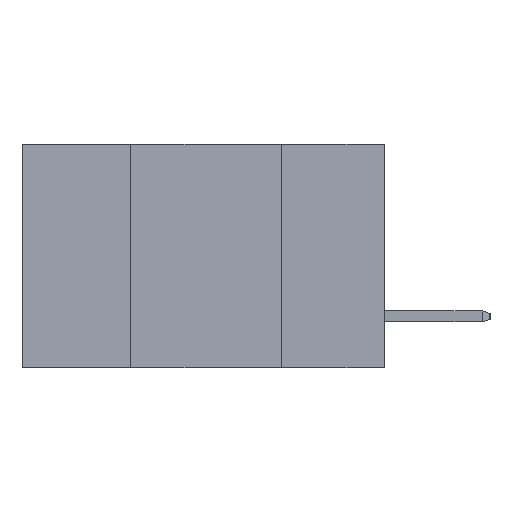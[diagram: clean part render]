
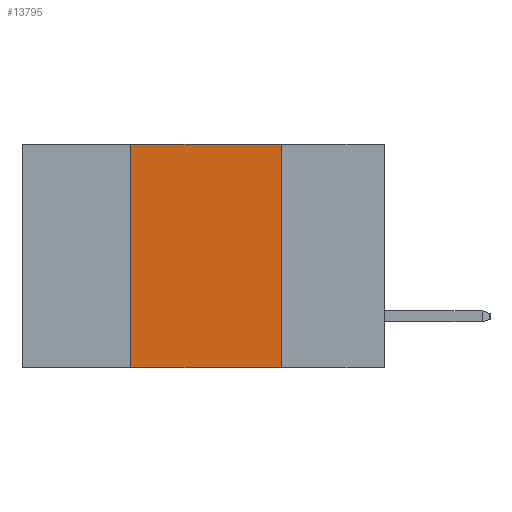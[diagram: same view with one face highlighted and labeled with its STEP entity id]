
A CAD part, left-side view. The second image highlights one B-rep face of the part: STEP entity #13795.
In plain terms, the highlighted planar face has unit normal (-1, 0, 0).
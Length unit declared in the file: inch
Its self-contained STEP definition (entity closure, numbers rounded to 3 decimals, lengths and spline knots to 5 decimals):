
#820 = CARTESIAN_POINT ( 'NONE',  ( 0., 0.42, 0. ) ) ;
#958 = DIRECTION ( 'NONE',  ( 0., 0., -1. ) ) ;
#1240 = AXIS2_PLACEMENT_3D ( 'NONE', #6806, #9732, #958 ) ;
#1403 = VERTEX_POINT ( 'NONE', #9511 ) ;
#3280 = ORIENTED_EDGE ( 'NONE', *, *, #6841, .F. ) ;
#3602 = FACE_OUTER_BOUND ( 'NONE', #16692, .T. ) ;
#4205 = CARTESIAN_POINT ( 'NONE',  ( 0., 0.42, 0. ) ) ;
#6280 = CARTESIAN_POINT ( 'NONE',  ( 0., 0.6, -0.37 ) ) ;
#6683 = ORIENTED_EDGE ( 'NONE', *, *, #8721, .F. ) ;
#6806 = CARTESIAN_POINT ( 'NONE',  ( 0., 0.6, 0. ) ) ;
#6841 = EDGE_CURVE ( 'NONE', #14572, #15960, #9867, .T. ) ;
#7154 = DIRECTION ( 'NONE',  ( 0., 0., -1. ) ) ;
#8253 = ORIENTED_EDGE ( 'NONE', *, *, #12579, .T. ) ;
#8721 = EDGE_CURVE ( 'NONE', #1403, #13756, #10246, .T. ) ;
#9443 = VECTOR ( 'NONE', #7154, 39.37008 ) ;
#9511 = CARTESIAN_POINT ( 'NONE',  ( 0., 0.42, -0.37 ) ) ;
#9732 = DIRECTION ( 'NONE',  ( 1., 0., 0. ) ) ;
#9867 = LINE ( 'NONE', #11359, #9443 ) ;
#10246 = LINE ( 'NONE', #4205, #13594 ) ;
#11359 = CARTESIAN_POINT ( 'NONE',  ( 0., 0.17, 0. ) ) ;
#12579 = EDGE_CURVE ( 'NONE', #1403, #15960, #14120, .T. ) ;
#12611 = EDGE_CURVE ( 'NONE', #13756, #14572, #13253, .T. ) ;
#12738 = DIRECTION ( 'NONE',  ( 0., 0., 1. ) ) ;
#12966 = CARTESIAN_POINT ( 'NONE',  ( 0., 0.17, 0. ) ) ;
#13253 = LINE ( 'NONE', #14201, #16493 ) ;
#13356 = CARTESIAN_POINT ( 'NONE',  ( 0., 0.17, -0.37 ) ) ;
#13594 = VECTOR ( 'NONE', #12738, 39.37008 ) ;
#13756 = VERTEX_POINT ( 'NONE', #820 ) ;
#13795 = ADVANCED_FACE ( 'NONE', ( #3602 ), #18049, .F. ) ;
#14120 = LINE ( 'NONE', #6280, #14560 ) ;
#14201 = CARTESIAN_POINT ( 'NONE',  ( 0., 0.6, 0. ) ) ;
#14560 = VECTOR ( 'NONE', #18190, 39.37008 ) ;
#14572 = VERTEX_POINT ( 'NONE', #12966 ) ;
#15586 = DIRECTION ( 'NONE',  ( 0., -1., 0. ) ) ;
#15960 = VERTEX_POINT ( 'NONE', #13356 ) ;
#16493 = VECTOR ( 'NONE', #15586, 39.37008 ) ;
#16692 = EDGE_LOOP ( 'NONE', ( #3280, #17432, #6683, #8253 ) ) ;
#17432 = ORIENTED_EDGE ( 'NONE', *, *, #12611, .F. ) ;
#18049 = PLANE ( 'NONE',  #1240 ) ;
#18190 = DIRECTION ( 'NONE',  ( 0., -1., 0. ) ) ;
